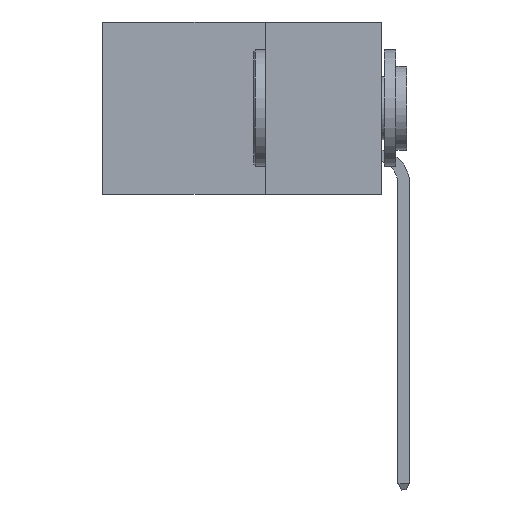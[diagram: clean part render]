
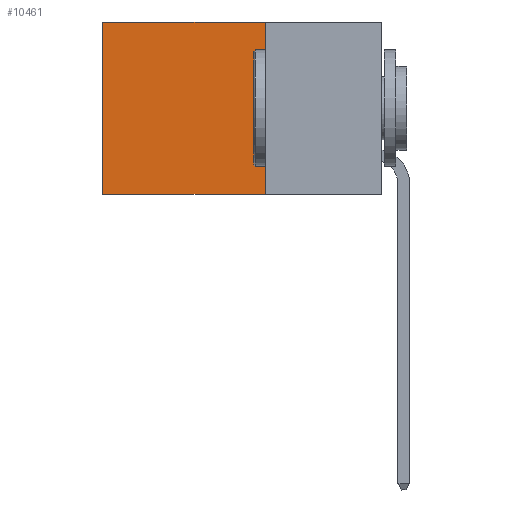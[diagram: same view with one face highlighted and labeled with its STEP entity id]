
A CAD part, left-side view. The second image highlights one B-rep face of the part: STEP entity #10461.
In plain terms, the highlighted planar face has unit normal (-1, 0, 0).
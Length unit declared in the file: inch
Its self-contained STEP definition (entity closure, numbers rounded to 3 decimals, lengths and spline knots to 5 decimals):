
#23 = ORIENTED_EDGE ( 'NONE', *, *, #7442, .T. ) ;
#146 = AXIS2_PLACEMENT_3D ( 'NONE', #6620, #6689, #7536 ) ;
#524 = DIRECTION ( 'NONE',  ( 0., 1., 0. ) ) ;
#575 = DIRECTION ( 'NONE',  ( 0., 1., 0. ) ) ;
#1736 = FACE_OUTER_BOUND ( 'NONE', #2349, .T. ) ;
#1948 = LINE ( 'NONE', #11309, #5252 ) ;
#2046 = LINE ( 'NONE', #9750, #7320 ) ;
#2106 = DIRECTION ( 'NONE',  ( 0., 0., -1. ) ) ;
#2200 = EDGE_CURVE ( 'NONE', #8090, #6150, #7036, .T. ) ;
#2349 = EDGE_LOOP ( 'NONE', ( #23, #10458, #8528, #4438 ) ) ;
#2403 = CARTESIAN_POINT ( 'NONE',  ( 0.2875, 0.25, 0. ) ) ;
#2781 = VECTOR ( 'NONE', #575, 39.37008 ) ;
#2918 = CARTESIAN_POINT ( 'NONE',  ( 0.2875, 0.6, -0.37 ) ) ;
#3362 = CARTESIAN_POINT ( 'NONE',  ( 0.2875, 0.6, 0. ) ) ;
#3764 = VECTOR ( 'NONE', #524, 39.37008 ) ;
#3963 = PLANE ( 'NONE',  #146 ) ;
#4412 = DIRECTION ( 'NONE',  ( 0., 0., -1. ) ) ;
#4438 = ORIENTED_EDGE ( 'NONE', *, *, #2200, .T. ) ;
#5252 = VECTOR ( 'NONE', #2106, 39.37008 ) ;
#6150 = VERTEX_POINT ( 'NONE', #3362 ) ;
#6620 = CARTESIAN_POINT ( 'NONE',  ( 0.2875, 0.25, 0. ) ) ;
#6689 = DIRECTION ( 'NONE',  ( 1., 0., 0. ) ) ;
#7036 = LINE ( 'NONE', #2403, #3764 ) ;
#7320 = VECTOR ( 'NONE', #4412, 39.37008 ) ;
#7442 = EDGE_CURVE ( 'NONE', #6150, #10779, #1948, .T. ) ;
#7536 = DIRECTION ( 'NONE',  ( 0., 0., -1. ) ) ;
#8090 = VERTEX_POINT ( 'NONE', #10248 ) ;
#8528 = ORIENTED_EDGE ( 'NONE', *, *, #9555, .F. ) ;
#9453 = EDGE_CURVE ( 'NONE', #9467, #10779, #11740, .T. ) ;
#9467 = VERTEX_POINT ( 'NONE', #10691 ) ;
#9555 = EDGE_CURVE ( 'NONE', #8090, #9467, #2046, .T. ) ;
#9750 = CARTESIAN_POINT ( 'NONE',  ( 0.2875, 0.25, 0. ) ) ;
#9787 = CARTESIAN_POINT ( 'NONE',  ( 0.2875, 0.25, -0.37 ) ) ;
#10248 = CARTESIAN_POINT ( 'NONE',  ( 0.2875, 0.25, 0. ) ) ;
#10458 = ORIENTED_EDGE ( 'NONE', *, *, #9453, .F. ) ;
#10461 = ADVANCED_FACE ( 'NONE', ( #1736 ), #3963, .F. ) ;
#10691 = CARTESIAN_POINT ( 'NONE',  ( 0.2875, 0.25, -0.37 ) ) ;
#10779 = VERTEX_POINT ( 'NONE', #2918 ) ;
#11309 = CARTESIAN_POINT ( 'NONE',  ( 0.2875, 0.6, 0. ) ) ;
#11740 = LINE ( 'NONE', #9787, #2781 ) ;
